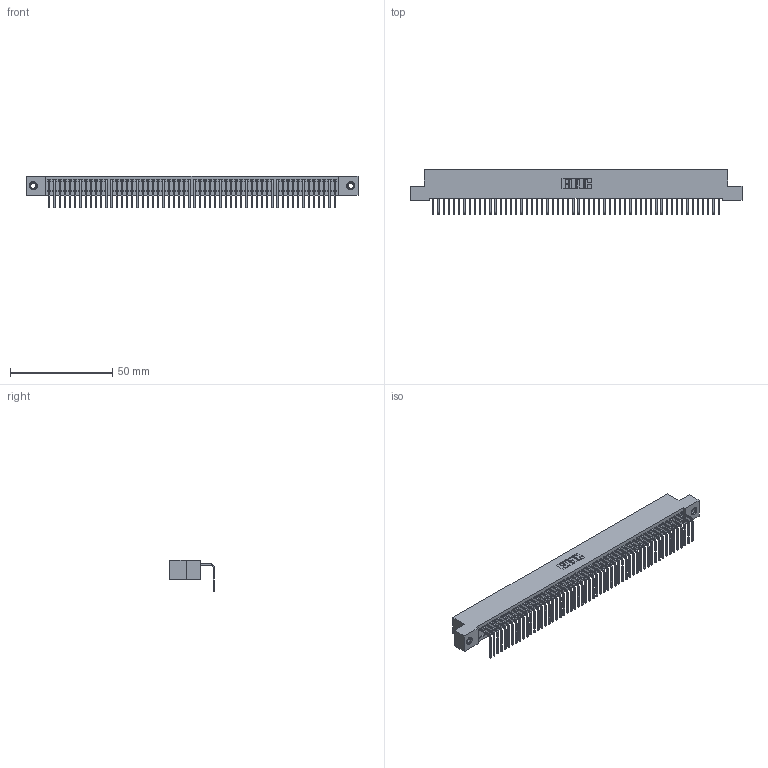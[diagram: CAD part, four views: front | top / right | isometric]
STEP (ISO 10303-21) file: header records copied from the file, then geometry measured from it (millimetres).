
FILE_DESCRIPTION (( 'STEP AP203' ), '1' );
FILE_NAME ('392-056-558-107.STEP', '2018-08-17T14:01:17', ( '' ), ( '' ), 'SwSTEP 2.0', 'SolidWorks 2016', '' );
FILE_SCHEMA (( 'CONFIG_CONTROL_DESIGN' ));
Length unit declared in the file: inch
Products named in the file (4): 342 Part_TI; 345-292-001_558 Tail - 2; 345-250-001_345-250-005-103; 392-056-558-107
Assembly tree (59 placements, depth 2):
  392-056-558-107
    342 Part_TI
    345-292-001_558 Tail - 2  x56
    345-250-001_345-250-005-103  x2
Bounding box: 162.56 x 21.91 x 15.62 mm (x, y, z)
Volume: 14478.7 mm3; surface area: 22614.6 mm2
Topology: 59 solids, 59 shells, 3530 faces, 10627 edges, 7002 vertices
Faces by surface type: plane 2562, cylinder 952, cone 12, torus 4
Entity records: 33562 total; most frequent: CARTESIAN_POINT 5769, ORIENTED_EDGE 5754, DIRECTION 4871, EDGE_CURVE 2877, LINE 2729, VECTOR 2729, VERTEX_POINT 1912, AXIS2_PLACEMENT_3D 1071
